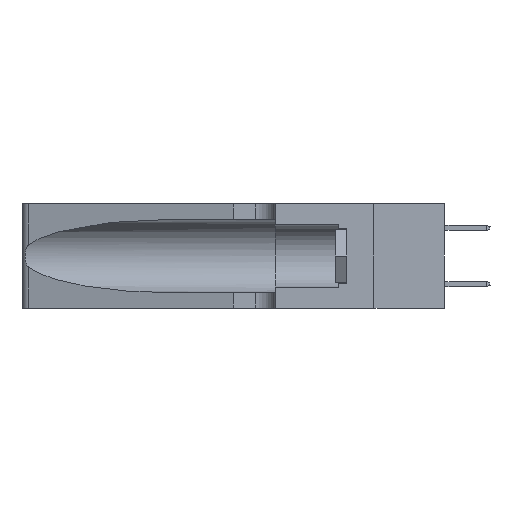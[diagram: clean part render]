
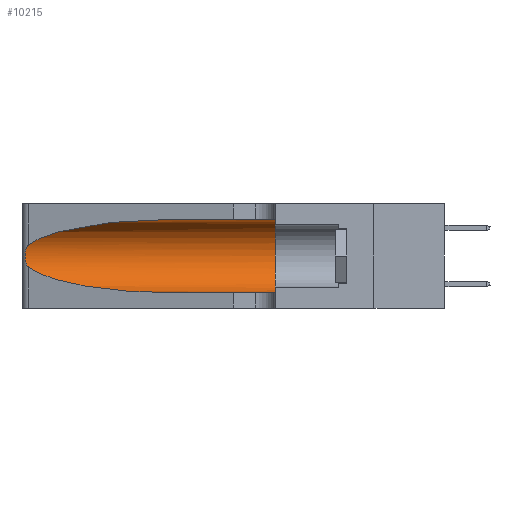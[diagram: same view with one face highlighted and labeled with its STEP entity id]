
A CAD part, left-side view. The second image highlights one B-rep face of the part: STEP entity #10215.
In plain terms, the highlighted cylindrical face has radius 3.308 mm (diameter 6.617 mm), a partial arc.
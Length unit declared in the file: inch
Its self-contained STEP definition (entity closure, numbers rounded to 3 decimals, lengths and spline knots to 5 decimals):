
#605 = VERTEX_POINT ( 'NONE', #9839 ) ;
#717 = CARTESIAN_POINT ( 'NONE',  ( 0.1305, 0.35, 0.31525 ) ) ;
#807 = FACE_OUTER_BOUND ( 'NONE', #7033, .T. ) ;
#870 = CARTESIAN_POINT ( 'NONE',  ( 0.18966, 0.96281, 0.05475 ) ) ;
#943 = CARTESIAN_POINT ( 'NONE',  ( 0.1305, 0.72297, 0.05475 ) ) ;
#1298 = CARTESIAN_POINT ( 'NONE',  ( 0.1305, 0.35, 0.05475 ) ) ;
#2024 = B_SPLINE_CURVE_WITH_KNOTS ( 'NONE', 3,
 ( #2570, #10324, #4134, #7195, #15164, #12128, #8737, #18451, #7265, #5759, #5462, #18598, #4062, #16776 ),
 .UNSPECIFIED., .F., .F.,
 ( 4, 2, 2, 2, 2, 2, 4 ),
 ( 0., 0.00027, 0.00053, 0.00107, 0.0016, 0.00187, 0.00214 ),
 .UNSPECIFIED. ) ;
#2053 = VERTEX_POINT ( 'NONE', #717 ) ;
#2076 = VECTOR ( 'NONE', #10432, 39.37008 ) ;
#2162 = CARTESIAN_POINT ( 'NONE',  ( 0.25487, 1.22718, 0.14631 ) ) ;
#2258 = ORIENTED_EDGE ( 'NONE', *, *, #19019, .T. ) ;
#2291 = ORIENTED_EDGE ( 'NONE', *, *, #11434, .F. ) ;
#2570 = CARTESIAN_POINT ( 'NONE',  ( 0.25487, 1.22718, 0.22369 ) ) ;
#2888 = VERTEX_POINT ( 'NONE', #4269 ) ;
#2919 = VERTEX_POINT ( 'NONE', #1298 ) ;
#3413 = CARTESIAN_POINT ( 'NONE',  ( 0.1305, 1.61858, 0.05475 ) ) ;
#3861 = VERTEX_POINT ( 'NONE', #15747 ) ;
#3981 =( BOUNDED_CURVE ( )  B_SPLINE_CURVE ( 3, ( #8944, #16987, #13801, #10815 ),
 .UNSPECIFIED., .F., .F. ) 
 B_SPLINE_CURVE_WITH_KNOTS ( ( 4, 4 ),
 ( 1.5708, 2.84003 ),
 .UNSPECIFIED. ) 
 CURVE ( )  GEOMETRIC_REPRESENTATION_ITEM ( )  RATIONAL_B_SPLINE_CURVE ( ( 1., 0.87, 0.87, 1. ) ) 
 REPRESENTATION_ITEM ( '' )  );
#4062 = CARTESIAN_POINT ( 'NONE',  ( 0.25555, 1.22993, 0.14849 ) ) ;
#4134 = CARTESIAN_POINT ( 'NONE',  ( 0.25639, 1.23184, 0.21858 ) ) ;
#4182 = DIRECTION ( 'NONE',  ( 0., 0., -1. ) ) ;
#4269 = CARTESIAN_POINT ( 'NONE',  ( 0.1305, 0.72297, 0.05475 ) ) ;
#4324 = AXIS2_PLACEMENT_3D ( 'NONE', #11969, #13792, #4182 ) ;
#5462 = CARTESIAN_POINT ( 'NONE',  ( 0.25789, 1.23486, 0.15765 ) ) ;
#5759 = CARTESIAN_POINT ( 'NONE',  ( 0.25856, 1.23593, 0.16098 ) ) ;
#7033 = EDGE_LOOP ( 'NONE', ( #2258, #18685, #9678, #7379, #2291, #9289 ) ) ;
#7195 = CARTESIAN_POINT ( 'NONE',  ( 0.25787, 1.23484, 0.2124 ) ) ;
#7265 = CARTESIAN_POINT ( 'NONE',  ( 0.26017, 1.23833, 0.17102 ) ) ;
#7379 = ORIENTED_EDGE ( 'NONE', *, *, #9945, .T. ) ;
#7864 = EDGE_CURVE ( 'NONE', #3861, #18076, #2024, .T. ) ;
#8094 = CARTESIAN_POINT ( 'NONE',  ( 0.1305, 0.35, 0.185 ) ) ;
#8737 = CARTESIAN_POINT ( 'NONE',  ( 0.26075, 1.23896, 0.19203 ) ) ;
#8944 = CARTESIAN_POINT ( 'NONE',  ( 0.1305, 0.72297, 0.31525 ) ) ;
#9289 = ORIENTED_EDGE ( 'NONE', *, *, #9720, .F. ) ;
#9678 = ORIENTED_EDGE ( 'NONE', *, *, #17290, .T. ) ;
#9720 = EDGE_CURVE ( 'NONE', #605, #2053, #11699, .T. ) ;
#9839 = CARTESIAN_POINT ( 'NONE',  ( 0.1305, 0.72297, 0.31525 ) ) ;
#9945 = EDGE_CURVE ( 'NONE', #2888, #2919, #13202, .T. ) ;
#9994 = DIRECTION ( 'NONE',  ( 0., -1., 0. ) ) ;
#10215 = ADVANCED_FACE ( 'NONE', ( #807 ), #19510, .F. ) ;
#10324 = CARTESIAN_POINT ( 'NONE',  ( 0.25555, 1.22994, 0.2215 ) ) ;
#10432 = DIRECTION ( 'NONE',  ( 0., -1., 0. ) ) ;
#10445 = CARTESIAN_POINT ( 'NONE',  ( 0.2373, 1.15595, 0.08982 ) ) ;
#10815 = CARTESIAN_POINT ( 'NONE',  ( 0.25487, 1.22718, 0.22369 ) ) ;
#11424 = DIRECTION ( 'NONE',  ( 0., 0., 1. ) ) ;
#11434 = EDGE_CURVE ( 'NONE', #2053, #2919, #12196, .T. ) ;
#11699 = LINE ( 'NONE', #15493, #2076 ) ;
#11760 =( BOUNDED_CURVE ( )  B_SPLINE_CURVE ( 3, ( #20067, #10445, #870, #943 ),
 .UNSPECIFIED., .F., .F. ) 
 B_SPLINE_CURVE_WITH_KNOTS ( ( 4, 4 ),
 ( 3.44316, 4.71239 ),
 .UNSPECIFIED. ) 
 CURVE ( )  GEOMETRIC_REPRESENTATION_ITEM ( )  RATIONAL_B_SPLINE_CURVE ( ( 1., 0.87, 0.87, 1. ) ) 
 REPRESENTATION_ITEM ( '' )  );
#11969 = CARTESIAN_POINT ( 'NONE',  ( 0.1305, 1.61858, 0.185 ) ) ;
#12128 = CARTESIAN_POINT ( 'NONE',  ( 0.26018, 1.23835, 0.19895 ) ) ;
#12196 = CIRCLE ( 'NONE', #13527, 0.13025 ) ;
#12732 = VECTOR ( 'NONE', #9994, 39.37008 ) ;
#13202 = LINE ( 'NONE', #3413, #12732 ) ;
#13527 = AXIS2_PLACEMENT_3D ( 'NONE', #8094, #19369, #11424 ) ;
#13792 = DIRECTION ( 'NONE',  ( 0., -1., 0. ) ) ;
#13801 = CARTESIAN_POINT ( 'NONE',  ( 0.2373, 1.15595, 0.28018 ) ) ;
#15164 = CARTESIAN_POINT ( 'NONE',  ( 0.25854, 1.2359, 0.20912 ) ) ;
#15493 = CARTESIAN_POINT ( 'NONE',  ( 0.1305, 1.61858, 0.31525 ) ) ;
#15747 = CARTESIAN_POINT ( 'NONE',  ( 0.25487, 1.22718, 0.22369 ) ) ;
#16776 = CARTESIAN_POINT ( 'NONE',  ( 0.25487, 1.22718, 0.14631 ) ) ;
#16987 = CARTESIAN_POINT ( 'NONE',  ( 0.18966, 0.96281, 0.31525 ) ) ;
#17290 = EDGE_CURVE ( 'NONE', #18076, #2888, #11760, .T. ) ;
#18076 = VERTEX_POINT ( 'NONE', #2162 ) ;
#18451 = CARTESIAN_POINT ( 'NONE',  ( 0.26075, 1.23896, 0.178 ) ) ;
#18598 = CARTESIAN_POINT ( 'NONE',  ( 0.25639, 1.23186, 0.15144 ) ) ;
#18685 = ORIENTED_EDGE ( 'NONE', *, *, #7864, .T. ) ;
#19019 = EDGE_CURVE ( 'NONE', #605, #3861, #3981, .T. ) ;
#19369 = DIRECTION ( 'NONE',  ( 0., 1., 0. ) ) ;
#19510 = CYLINDRICAL_SURFACE ( 'NONE', #4324, 0.13025 ) ;
#20067 = CARTESIAN_POINT ( 'NONE',  ( 0.25487, 1.22718, 0.14631 ) ) ;
